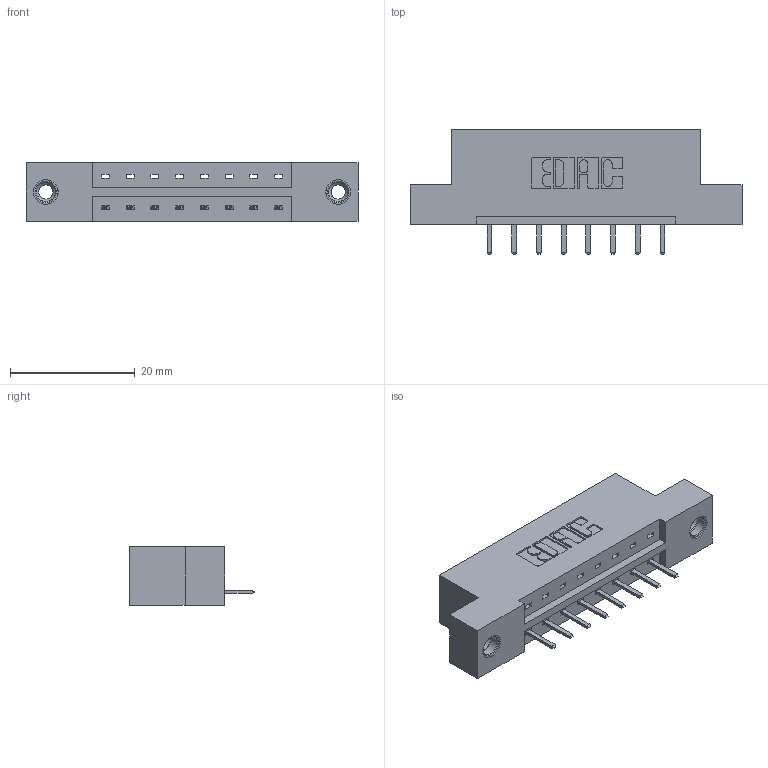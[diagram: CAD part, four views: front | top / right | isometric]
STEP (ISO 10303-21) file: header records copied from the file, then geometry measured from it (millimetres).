
FILE_DESCRIPTION (( 'STEP AP203' ), '1' );
FILE_NAME ('333-008-520-108.STEP', '2018-07-31T21:54:32', ( '' ), ( '' ), 'SwSTEP 2.0', 'SolidWorks 2016', '' );
FILE_SCHEMA (( 'CONFIG_CONTROL_DESIGN' ));
Length unit declared in the file: inch
Products named in the file (4): 345-292-001_345-293-120; 345-250-001_345-250-003-102; 333-008-520-108; 333 Part_Flush - .156 Dia - TI
Assembly tree (11 placements, depth 2):
  333-008-520-108
    333 Part_Flush - .156 Dia - TI
    345-292-001_345-293-120  x8
    345-250-001_345-250-003-102  x2
Bounding box: 53.24 x 20.02 x 9.4 mm (x, y, z)
Volume: 5035.4 mm3; surface area: 5170.7 mm2
Topology: 11 solids, 11 shells, 670 faces, 1919 edges, 1250 vertices
Faces by surface type: plane 454, cylinder 200, cone 12, torus 4
Entity records: 10588 total; most frequent: CARTESIAN_POINT 1825, ORIENTED_EDGE 1750, DIRECTION 1629, EDGE_CURVE 875, LINE 723, VECTOR 723, VERTEX_POINT 576, AXIS2_PLACEMENT_3D 453
